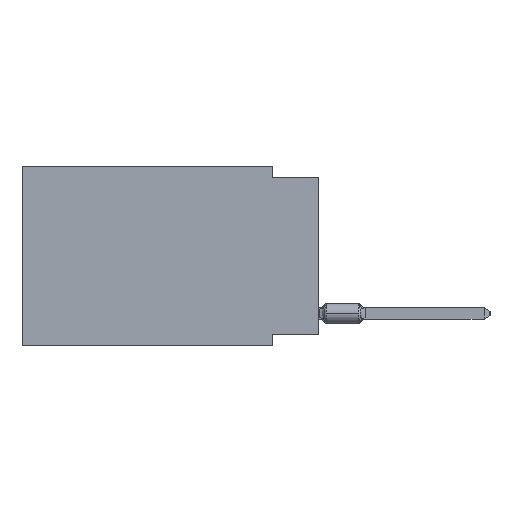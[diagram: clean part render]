
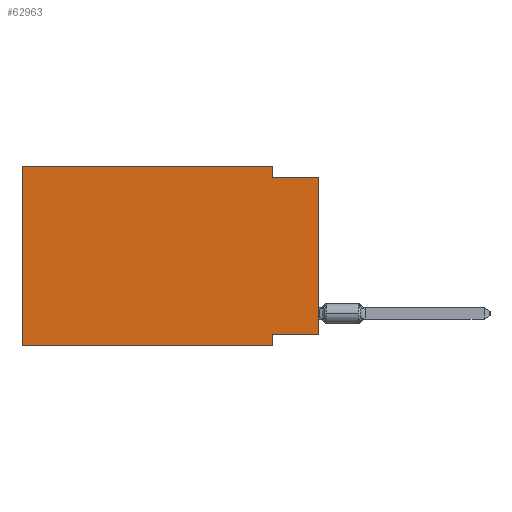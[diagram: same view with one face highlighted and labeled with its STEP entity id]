
A CAD part, left-side view. The second image highlights one B-rep face of the part: STEP entity #62963.
In plain terms, the highlighted planar face has unit normal (-1, 0, 0).
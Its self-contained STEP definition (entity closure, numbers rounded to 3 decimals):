
#2668 = CARTESIAN_POINT ( 'NONE',  ( 0., 16.383, -9.906 ) ) ;
#4073 = EDGE_CURVE ( 'NONE', #38519, #14305, #68665, .T. ) ;
#4814 = DIRECTION ( 'NONE',  ( 0., -1., 0. ) ) ;
#5152 = CARTESIAN_POINT ( 'NONE',  ( 0., 16.383, 0. ) ) ;
#5209 = ORIENTED_EDGE ( 'NONE', *, *, #4073, .F. ) ;
#5363 = EDGE_LOOP ( 'NONE', ( #7733, #59715, #31702, #5209, #48211, #54138, #57644, #32661 ) ) ;
#5780 = DIRECTION ( 'NONE',  ( 0., 0., -1. ) ) ;
#6861 = VECTOR ( 'NONE', #55581, 1000. ) ;
#7651 = DIRECTION ( 'NONE',  ( 0., -1., 0. ) ) ;
#7733 = ORIENTED_EDGE ( 'NONE', *, *, #51295, .T. ) ;
#8212 = DIRECTION ( 'NONE',  ( 0., 1., 0. ) ) ;
#10884 = CARTESIAN_POINT ( 'NONE',  ( 0., 0., -0.635 ) ) ;
#11225 = VERTEX_POINT ( 'NONE', #33729 ) ;
#11589 = VECTOR ( 'NONE', #15563, 1000. ) ;
#11725 = VECTOR ( 'NONE', #19761, 1000. ) ;
#12196 = EDGE_CURVE ( 'NONE', #40811, #55658, #31048, .T. ) ;
#14105 = LINE ( 'NONE', #32656, #11725 ) ;
#14305 = VERTEX_POINT ( 'NONE', #33726 ) ;
#15165 = LINE ( 'NONE', #51900, #11589 ) ;
#15563 = DIRECTION ( 'NONE',  ( 0., 0., 1. ) ) ;
#19761 = DIRECTION ( 'NONE',  ( 0., 0., -1. ) ) ;
#20363 = CARTESIAN_POINT ( 'NONE',  ( 0., 2.54, -9.906 ) ) ;
#21152 = CARTESIAN_POINT ( 'NONE',  ( 0., 0., -9.271 ) ) ;
#22197 = CARTESIAN_POINT ( 'NONE',  ( 0., 2.54, -0.635 ) ) ;
#22561 = DIRECTION ( 'NONE',  ( 1., 0., 0. ) ) ;
#23456 = VECTOR ( 'NONE', #8212, 1000. ) ;
#23965 = CARTESIAN_POINT ( 'NONE',  ( 0., 2.54, -9.906 ) ) ;
#24927 = CARTESIAN_POINT ( 'NONE',  ( 0., 16.383, 0. ) ) ;
#31048 = LINE ( 'NONE', #10884, #72667 ) ;
#31702 = ORIENTED_EDGE ( 'NONE', *, *, #65083, .F. ) ;
#32656 = CARTESIAN_POINT ( 'NONE',  ( 0., 2.54, 0. ) ) ;
#32661 = ORIENTED_EDGE ( 'NONE', *, *, #40055, .F. ) ;
#33726 = CARTESIAN_POINT ( 'NONE',  ( 0., 2.54, 0. ) ) ;
#33729 = CARTESIAN_POINT ( 'NONE',  ( 0., 2.54, -9.271 ) ) ;
#33778 = EDGE_CURVE ( 'NONE', #11225, #37905, #67201, .T. ) ;
#37905 = VERTEX_POINT ( 'NONE', #20363 ) ;
#38519 = VERTEX_POINT ( 'NONE', #24927 ) ;
#40055 = EDGE_CURVE ( 'NONE', #59809, #11225, #70833, .T. ) ;
#40811 = VERTEX_POINT ( 'NONE', #22197 ) ;
#42032 = DIRECTION ( 'NONE',  ( 0., -1., 0. ) ) ;
#45611 = CARTESIAN_POINT ( 'NONE',  ( 0., 16.383, 0. ) ) ;
#47701 = CARTESIAN_POINT ( 'NONE',  ( 0., 16.383, -9.906 ) ) ;
#48211 = ORIENTED_EDGE ( 'NONE', *, *, #70371, .F. ) ;
#48988 = EDGE_CURVE ( 'NONE', #73912, #37905, #67089, .T. ) ;
#51295 = EDGE_CURVE ( 'NONE', #59809, #55658, #15165, .T. ) ;
#51900 = CARTESIAN_POINT ( 'NONE',  ( 0., 0., 0. ) ) ;
#54138 = ORIENTED_EDGE ( 'NONE', *, *, #48988, .T. ) ;
#54741 = VECTOR ( 'NONE', #7651, 1000. ) ;
#55581 = DIRECTION ( 'NONE',  ( 0., 0., 1. ) ) ;
#55658 = VERTEX_POINT ( 'NONE', #65454 ) ;
#57644 = ORIENTED_EDGE ( 'NONE', *, *, #33778, .F. ) ;
#59715 = ORIENTED_EDGE ( 'NONE', *, *, #12196, .F. ) ;
#59809 = VERTEX_POINT ( 'NONE', #64965 ) ;
#60514 = FACE_OUTER_BOUND ( 'NONE', #5363, .T. ) ;
#62963 = ADVANCED_FACE ( 'NONE', ( #60514 ), #79485, .F. ) ;
#64965 = CARTESIAN_POINT ( 'NONE',  ( 0., 0., -9.271 ) ) ;
#65083 = EDGE_CURVE ( 'NONE', #14305, #40811, #14105, .T. ) ;
#65454 = CARTESIAN_POINT ( 'NONE',  ( 0., 0., -0.635 ) ) ;
#67089 = LINE ( 'NONE', #47701, #78452 ) ;
#67201 = LINE ( 'NONE', #23965, #75254 ) ;
#67705 = LINE ( 'NONE', #79818, #6861 ) ;
#68665 = LINE ( 'NONE', #45611, #54741 ) ;
#70371 = EDGE_CURVE ( 'NONE', #73912, #38519, #67705, .T. ) ;
#70833 = LINE ( 'NONE', #21152, #23456 ) ;
#72667 = VECTOR ( 'NONE', #4814, 1000. ) ;
#73912 = VERTEX_POINT ( 'NONE', #2668 ) ;
#74711 = AXIS2_PLACEMENT_3D ( 'NONE', #5152, #22561, #79083 ) ;
#75254 = VECTOR ( 'NONE', #5780, 1000. ) ;
#78452 = VECTOR ( 'NONE', #42032, 1000. ) ;
#79083 = DIRECTION ( 'NONE',  ( 0., 0., -1. ) ) ;
#79485 = PLANE ( 'NONE',  #74711 ) ;
#79818 = CARTESIAN_POINT ( 'NONE',  ( 0., 16.383, 0. ) ) ;
